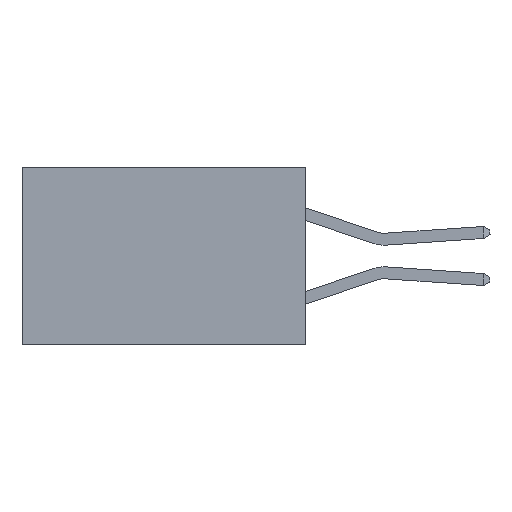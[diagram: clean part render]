
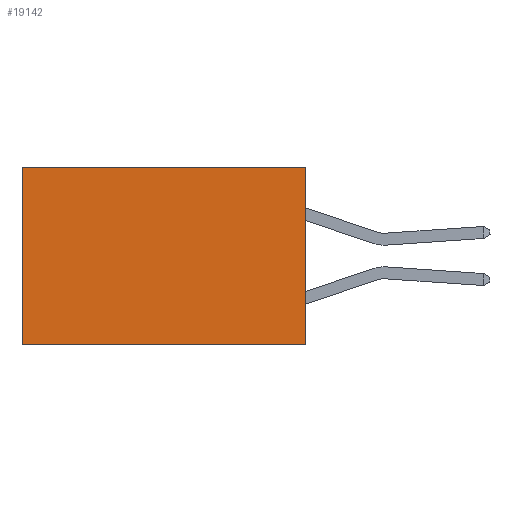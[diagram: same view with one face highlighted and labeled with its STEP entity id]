
A CAD part, left-side view. The second image highlights one B-rep face of the part: STEP entity #19142.
In plain terms, the highlighted planar face has unit normal (-1, 0, 0).
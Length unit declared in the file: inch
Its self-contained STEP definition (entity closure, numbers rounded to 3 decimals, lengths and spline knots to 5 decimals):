
#1031 = VECTOR ( 'NONE', #6118, 39.37008 ) ;
#1188 = EDGE_CURVE ( 'NONE', #26308, #3982, #26146, .T. ) ;
#1381 = LINE ( 'NONE', #17088, #7176 ) ;
#1701 = LINE ( 'NONE', #27004, #1031 ) ;
#2290 = CARTESIAN_POINT ( 'NONE',  ( 0.277, 0.59, -0.37 ) ) ;
#2325 = DIRECTION ( 'NONE',  ( 0., 0., -1. ) ) ;
#2640 = DIRECTION ( 'NONE',  ( 0., 0., -1. ) ) ;
#2836 = VERTEX_POINT ( 'NONE', #16608 ) ;
#3982 = VERTEX_POINT ( 'NONE', #22934 ) ;
#4480 = VECTOR ( 'NONE', #2325, 39.37008 ) ;
#4662 = ORIENTED_EDGE ( 'NONE', *, *, #7743, .T. ) ;
#6118 = DIRECTION ( 'NONE',  ( 0., 0., -1. ) ) ;
#6429 = VECTOR ( 'NONE', #12087, 39.37008 ) ;
#7176 = VECTOR ( 'NONE', #27194, 39.37008 ) ;
#7609 = VERTEX_POINT ( 'NONE', #11783 ) ;
#7743 = EDGE_CURVE ( 'NONE', #2836, #26308, #11207, .T. ) ;
#8428 = CARTESIAN_POINT ( 'NONE',  ( 0.277, 0.59, 0. ) ) ;
#9112 = CARTESIAN_POINT ( 'NONE',  ( 0.277, 0., -0.37 ) ) ;
#10333 = EDGE_CURVE ( 'NONE', #2836, #7609, #1701, .T. ) ;
#11207 = LINE ( 'NONE', #12059, #6429 ) ;
#11731 = AXIS2_PLACEMENT_3D ( 'NONE', #9112, #15556, #2640 ) ;
#11783 = CARTESIAN_POINT ( 'NONE',  ( 0.277, 0., -0.37 ) ) ;
#12059 = CARTESIAN_POINT ( 'NONE',  ( 0.277, 0., 0. ) ) ;
#12087 = DIRECTION ( 'NONE',  ( 0., 1., 0. ) ) ;
#15446 = ORIENTED_EDGE ( 'NONE', *, *, #10333, .F. ) ;
#15556 = DIRECTION ( 'NONE',  ( 1., 0., 0. ) ) ;
#16608 = CARTESIAN_POINT ( 'NONE',  ( 0.277, 0., 0. ) ) ;
#17088 = CARTESIAN_POINT ( 'NONE',  ( 0.277, 0., -0.37 ) ) ;
#18966 = ORIENTED_EDGE ( 'NONE', *, *, #1188, .T. ) ;
#19138 = FACE_OUTER_BOUND ( 'NONE', #19435, .T. ) ;
#19142 = ADVANCED_FACE ( 'NONE', ( #19138 ), #25746, .F. ) ;
#19435 = EDGE_LOOP ( 'NONE', ( #18966, #25682, #15446, #4662 ) ) ;
#19647 = EDGE_CURVE ( 'NONE', #7609, #3982, #1381, .T. ) ;
#22934 = CARTESIAN_POINT ( 'NONE',  ( 0.277, 0.59, -0.37 ) ) ;
#25682 = ORIENTED_EDGE ( 'NONE', *, *, #19647, .F. ) ;
#25746 = PLANE ( 'NONE',  #11731 ) ;
#26146 = LINE ( 'NONE', #2290, #4480 ) ;
#26308 = VERTEX_POINT ( 'NONE', #8428 ) ;
#27004 = CARTESIAN_POINT ( 'NONE',  ( 0.277, 0., -0.37 ) ) ;
#27194 = DIRECTION ( 'NONE',  ( 0., 1., 0. ) ) ;
